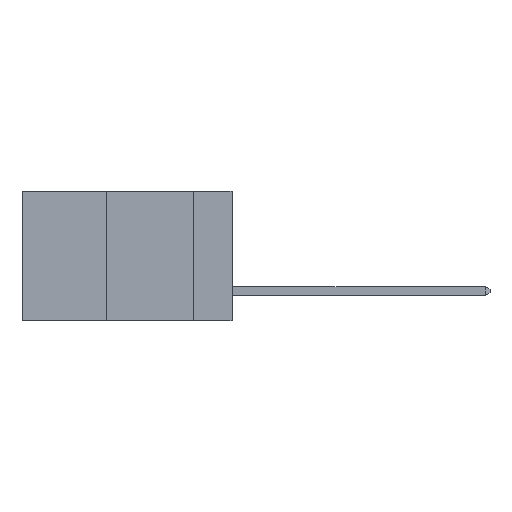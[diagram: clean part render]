
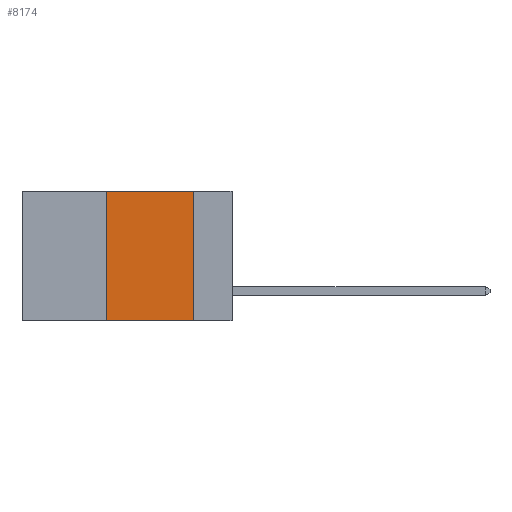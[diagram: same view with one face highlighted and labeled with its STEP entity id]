
A CAD part, left-side view. The second image highlights one B-rep face of the part: STEP entity #8174.
In plain terms, the highlighted planar face has unit normal (-1, 0, 0).
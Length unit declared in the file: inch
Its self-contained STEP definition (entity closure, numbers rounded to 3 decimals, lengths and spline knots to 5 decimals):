
#1748 = VERTEX_POINT ( 'NONE', #16328 ) ;
#1975 = DIRECTION ( 'NONE',  ( 0., 0., -1. ) ) ;
#2512 = PLANE ( 'NONE',  #5410 ) ;
#3776 = VECTOR ( 'NONE', #20282, 39.37008 ) ;
#4490 = DIRECTION ( 'NONE',  ( 0., 0., -1. ) ) ;
#4491 = CARTESIAN_POINT ( 'NONE',  ( 0., 0.6, 0. ) ) ;
#5154 = LINE ( 'NONE', #9480, #9034 ) ;
#5410 = AXIS2_PLACEMENT_3D ( 'NONE', #15757, #15837, #4490 ) ;
#5498 = CARTESIAN_POINT ( 'NONE',  ( 0., 0.11, 0. ) ) ;
#6413 = ORIENTED_EDGE ( 'NONE', *, *, #23009, .T. ) ;
#8174 = ADVANCED_FACE ( 'NONE', ( #14469 ), #2512, .F. ) ;
#8838 = VECTOR ( 'NONE', #15840, 39.37008 ) ;
#9034 = VECTOR ( 'NONE', #11370, 39.37008 ) ;
#9480 = CARTESIAN_POINT ( 'NONE',  ( 0., 0.36, 0. ) ) ;
#10285 = ORIENTED_EDGE ( 'NONE', *, *, #23483, .F. ) ;
#10425 = CARTESIAN_POINT ( 'NONE',  ( 0., 0.36, -0.37 ) ) ;
#11017 = EDGE_LOOP ( 'NONE', ( #19179, #10285, #15317, #6413 ) ) ;
#11370 = DIRECTION ( 'NONE',  ( 0., 0., 1. ) ) ;
#14469 = FACE_OUTER_BOUND ( 'NONE', #11017, .T. ) ;
#15317 = ORIENTED_EDGE ( 'NONE', *, *, #16150, .F. ) ;
#15341 = CARTESIAN_POINT ( 'NONE',  ( 0., 0.11, 0. ) ) ;
#15757 = CARTESIAN_POINT ( 'NONE',  ( 0., 0.6, 0. ) ) ;
#15801 = VECTOR ( 'NONE', #1975, 39.37008 ) ;
#15837 = DIRECTION ( 'NONE',  ( 1., 0., 0. ) ) ;
#15840 = DIRECTION ( 'NONE',  ( 0., -1., 0. ) ) ;
#16150 = EDGE_CURVE ( 'NONE', #17475, #24015, #5154, .T. ) ;
#16328 = CARTESIAN_POINT ( 'NONE',  ( 0., 0.11, -0.37 ) ) ;
#16526 = EDGE_CURVE ( 'NONE', #18245, #1748, #20864, .T. ) ;
#17475 = VERTEX_POINT ( 'NONE', #10425 ) ;
#17841 = CARTESIAN_POINT ( 'NONE',  ( 0., 0.36, 0. ) ) ;
#18245 = VERTEX_POINT ( 'NONE', #5498 ) ;
#18909 = LINE ( 'NONE', #4491, #8838 ) ;
#18928 = LINE ( 'NONE', #24031, #3776 ) ;
#19179 = ORIENTED_EDGE ( 'NONE', *, *, #16526, .F. ) ;
#20282 = DIRECTION ( 'NONE',  ( 0., -1., 0. ) ) ;
#20864 = LINE ( 'NONE', #15341, #15801 ) ;
#23009 = EDGE_CURVE ( 'NONE', #17475, #1748, #18928, .T. ) ;
#23483 = EDGE_CURVE ( 'NONE', #24015, #18245, #18909, .T. ) ;
#24015 = VERTEX_POINT ( 'NONE', #17841 ) ;
#24031 = CARTESIAN_POINT ( 'NONE',  ( 0., 0.6, -0.37 ) ) ;
